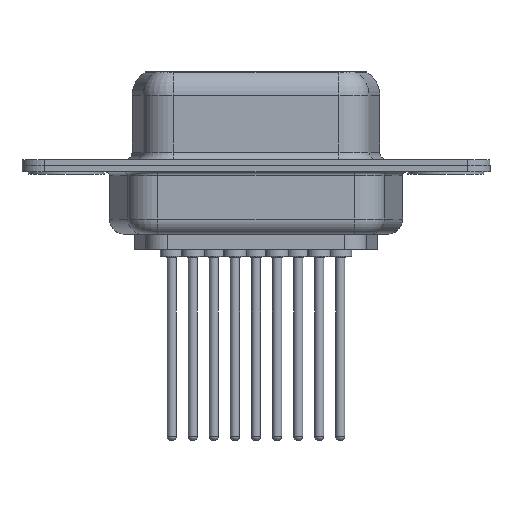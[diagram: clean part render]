
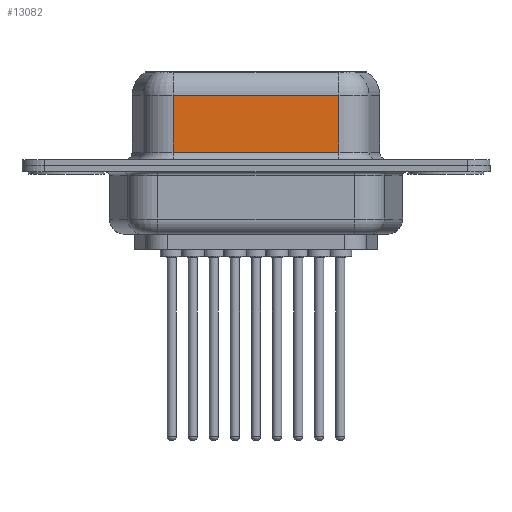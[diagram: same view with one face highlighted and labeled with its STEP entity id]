
A CAD part, front view. The second image highlights one B-rep face of the part: STEP entity #13082.
In plain terms, the highlighted planar face has unit normal (0, -1, 0).
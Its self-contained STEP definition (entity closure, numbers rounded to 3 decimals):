
#203 = DIRECTION ( 'NONE',  ( 0., 0., -1. ) ) ;
#851 = EDGE_CURVE ( 'NONE', #10438, #9101, #1573, .T. ) ;
#1313 = EDGE_LOOP ( 'NONE', ( #12177, #12841, #2373, #9665 ) ) ;
#1573 = LINE ( 'NONE', #10012, #8549 ) ;
#2373 = ORIENTED_EDGE ( 'NONE', *, *, #8814, .T. ) ;
#2784 = CARTESIAN_POINT ( 'NONE',  ( 7.038, -3.95, 6.4 ) ) ;
#2900 = FACE_OUTER_BOUND ( 'NONE', #1313, .T. ) ;
#3925 = DIRECTION ( 'NONE',  ( 0., 0., 1. ) ) ;
#4160 = AXIS2_PLACEMENT_3D ( 'NONE', #12499, #7116, #3925 ) ;
#4436 = CARTESIAN_POINT ( 'NONE',  ( 17.962, -3.95, 4.65 ) ) ;
#5030 = CARTESIAN_POINT ( 'NONE',  ( 7.038, -3.95, 0.9 ) ) ;
#5980 = LINE ( 'NONE', #2784, #10053 ) ;
#6159 = PLANE ( 'NONE',  #4160 ) ;
#7116 = DIRECTION ( 'NONE',  ( 0., 1., 0. ) ) ;
#7564 = LINE ( 'NONE', #4436, #8511 ) ;
#7677 = CARTESIAN_POINT ( 'NONE',  ( 7.038, -3.95, 4.65 ) ) ;
#7851 = LINE ( 'NONE', #13091, #9150 ) ;
#7873 = EDGE_CURVE ( 'NONE', #12670, #9101, #7851, .T. ) ;
#8511 = VECTOR ( 'NONE', #8802, 1000. ) ;
#8549 = VECTOR ( 'NONE', #13228, 1000. ) ;
#8802 = DIRECTION ( 'NONE',  ( -1., 0., 0. ) ) ;
#8814 = EDGE_CURVE ( 'NONE', #9553, #10438, #5980, .T. ) ;
#8987 = EDGE_CURVE ( 'NONE', #12670, #9553, #7564, .T. ) ;
#9101 = VERTEX_POINT ( 'NONE', #10938 ) ;
#9150 = VECTOR ( 'NONE', #203, 1000. ) ;
#9168 = CARTESIAN_POINT ( 'NONE',  ( 17.962, -3.95, 4.65 ) ) ;
#9553 = VERTEX_POINT ( 'NONE', #7677 ) ;
#9665 = ORIENTED_EDGE ( 'NONE', *, *, #851, .T. ) ;
#10012 = CARTESIAN_POINT ( 'NONE',  ( 17.962, -3.95, 0.9 ) ) ;
#10053 = VECTOR ( 'NONE', #13415, 1000. ) ;
#10438 = VERTEX_POINT ( 'NONE', #5030 ) ;
#10938 = CARTESIAN_POINT ( 'NONE',  ( 17.962, -3.95, 0.9 ) ) ;
#12177 = ORIENTED_EDGE ( 'NONE', *, *, #7873, .F. ) ;
#12499 = CARTESIAN_POINT ( 'NONE',  ( 17.962, -3.95, 6.4 ) ) ;
#12670 = VERTEX_POINT ( 'NONE', #9168 ) ;
#12841 = ORIENTED_EDGE ( 'NONE', *, *, #8987, .T. ) ;
#13082 = ADVANCED_FACE ( 'NONE', ( #2900 ), #6159, .F. ) ;
#13091 = CARTESIAN_POINT ( 'NONE',  ( 17.962, -3.95, 6.4 ) ) ;
#13228 = DIRECTION ( 'NONE',  ( 1., 0., 0. ) ) ;
#13415 = DIRECTION ( 'NONE',  ( 0., 0., -1. ) ) ;
